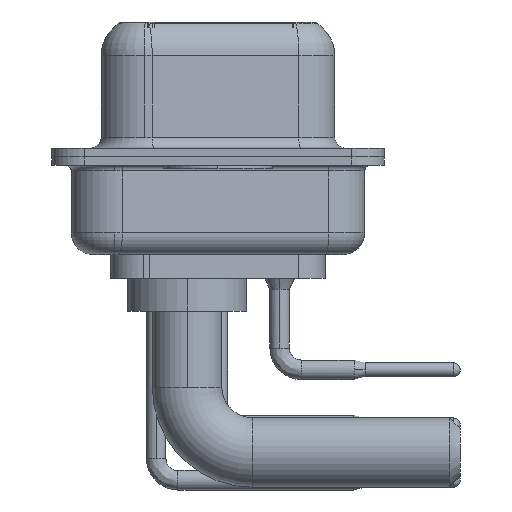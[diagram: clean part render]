
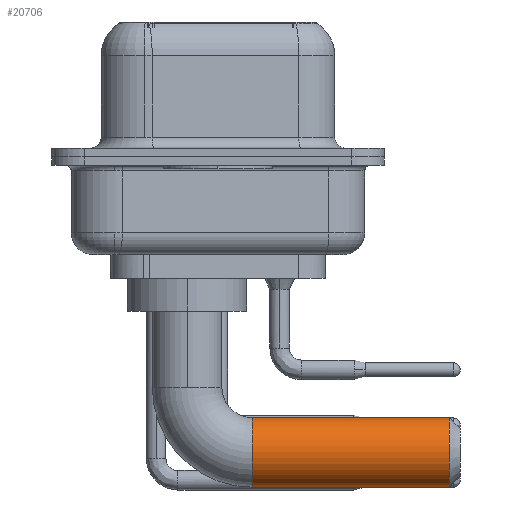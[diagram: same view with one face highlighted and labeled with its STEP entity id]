
A CAD part, left-side view. The second image highlights one B-rep face of the part: STEP entity #20706.
In plain terms, the highlighted cylindrical face has radius 1.6 mm (diameter 3.2 mm), a partial arc.
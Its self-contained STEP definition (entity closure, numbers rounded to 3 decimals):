
#517 = CARTESIAN_POINT ( 'NONE',  ( 0., -12.07, -4.9 ) ) ;
#543 = DIRECTION ( 'NONE',  ( -1., 0., 0. ) ) ;
#696 = CARTESIAN_POINT ( 'NONE',  ( 0., -3., -6.5 ) ) ;
#1028 = CARTESIAN_POINT ( 'NONE',  ( 0., -3., -8.1 ) ) ;
#1132 = VECTOR ( 'NONE', #8485, 1000. ) ;
#2072 = VERTEX_POINT ( 'NONE', #2639 ) ;
#2639 = CARTESIAN_POINT ( 'NONE',  ( 0., -12.07, -8.1 ) ) ;
#2915 = DIRECTION ( 'NONE',  ( 0., -1., 0. ) ) ;
#3194 = VERTEX_POINT ( 'NONE', #16647 ) ;
#5540 = ORIENTED_EDGE ( 'NONE', *, *, #17622, .F. ) ;
#5713 = LINE ( 'NONE', #1028, #13710 ) ;
#6574 = CYLINDRICAL_SURFACE ( 'NONE', #15163, 1.6 ) ;
#7443 = ORIENTED_EDGE ( 'NONE', *, *, #21500, .T. ) ;
#7890 = EDGE_LOOP ( 'NONE', ( #5540, #26699, #7443, #8998 ) ) ;
#8181 = CARTESIAN_POINT ( 'NONE',  ( 0., -3., -4.9 ) ) ;
#8485 = DIRECTION ( 'NONE',  ( 0., -1., 0. ) ) ;
#8735 = DIRECTION ( 'NONE',  ( 0., -1., 0. ) ) ;
#8998 = ORIENTED_EDGE ( 'NONE', *, *, #27288, .T. ) ;
#10499 = LINE ( 'NONE', #8181, #1132 ) ;
#10894 = FACE_OUTER_BOUND ( 'NONE', #7890, .T. ) ;
#11142 = EDGE_CURVE ( 'NONE', #3194, #12206, #23756, .T. ) ;
#12206 = VERTEX_POINT ( 'NONE', #14489 ) ;
#13710 = VECTOR ( 'NONE', #29330, 1000. ) ;
#14489 = CARTESIAN_POINT ( 'NONE',  ( 0., -3., -8.1 ) ) ;
#15163 = AXIS2_PLACEMENT_3D ( 'NONE', #20532, #8735, #25230 ) ;
#16385 = CARTESIAN_POINT ( 'NONE',  ( 0., -12.07, -6.5 ) ) ;
#16534 = DIRECTION ( 'NONE',  ( 0., 1., 0. ) ) ;
#16647 = CARTESIAN_POINT ( 'NONE',  ( 0., -3., -4.9 ) ) ;
#17622 = EDGE_CURVE ( 'NONE', #3194, #19609, #10499, .T. ) ;
#18288 = AXIS2_PLACEMENT_3D ( 'NONE', #696, #2915, #543 ) ;
#19609 = VERTEX_POINT ( 'NONE', #517 ) ;
#20532 = CARTESIAN_POINT ( 'NONE',  ( 0., -3., -6.5 ) ) ;
#20706 = ADVANCED_FACE ( 'NONE', ( #10894 ), #6574, .T. ) ;
#21500 = EDGE_CURVE ( 'NONE', #12206, #2072, #5713, .T. ) ;
#22447 = CIRCLE ( 'NONE', #29918, 1.6 ) ;
#23756 = CIRCLE ( 'NONE', #18288, 1.6 ) ;
#25230 = DIRECTION ( 'NONE',  ( 0., 0., -1. ) ) ;
#26052 = DIRECTION ( 'NONE',  ( 0., 0., -1. ) ) ;
#26699 = ORIENTED_EDGE ( 'NONE', *, *, #11142, .T. ) ;
#27288 = EDGE_CURVE ( 'NONE', #2072, #19609, #22447, .T. ) ;
#29330 = DIRECTION ( 'NONE',  ( 0., -1., 0. ) ) ;
#29918 = AXIS2_PLACEMENT_3D ( 'NONE', #16385, #16534, #26052 ) ;
